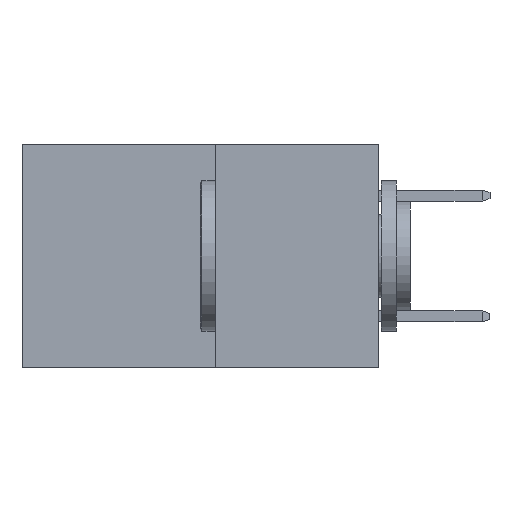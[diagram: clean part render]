
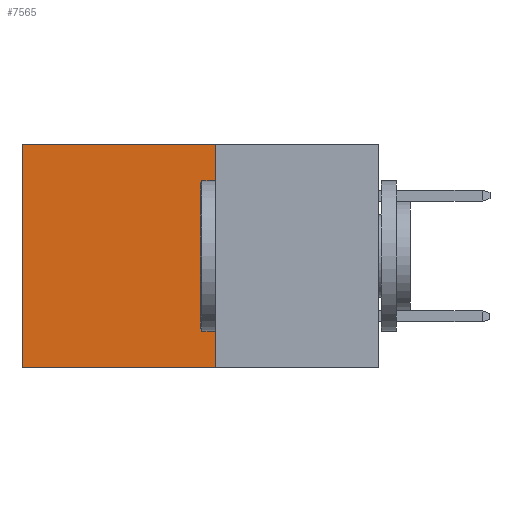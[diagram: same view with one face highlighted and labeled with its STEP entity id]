
A CAD part, left-side view. The second image highlights one B-rep face of the part: STEP entity #7565.
In plain terms, the highlighted planar face has unit normal (-1, 0, 0).
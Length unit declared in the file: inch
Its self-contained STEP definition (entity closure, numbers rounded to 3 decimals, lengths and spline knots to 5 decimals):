
#312 = AXIS2_PLACEMENT_3D ( 'NONE', #6959, #4473, #389 ) ;
#389 = DIRECTION ( 'NONE',  ( 0., 0., -1. ) ) ;
#523 = CARTESIAN_POINT ( 'NONE',  ( 0.277, 0.27, -0.37 ) ) ;
#697 = LINE ( 'NONE', #523, #2576 ) ;
#932 = DIRECTION ( 'NONE',  ( 0., 1., 0. ) ) ;
#1072 = ORIENTED_EDGE ( 'NONE', *, *, #3635, .F. ) ;
#1086 = CARTESIAN_POINT ( 'NONE',  ( 0.277, 0.27, -0.37 ) ) ;
#1194 = FACE_OUTER_BOUND ( 'NONE', #4344, .T. ) ;
#1295 = DIRECTION ( 'NONE',  ( 0., 0., -1. ) ) ;
#1376 = LINE ( 'NONE', #7771, #7960 ) ;
#2576 = VECTOR ( 'NONE', #1295, 39.37008 ) ;
#3232 = LINE ( 'NONE', #7819, #6601 ) ;
#3635 = EDGE_CURVE ( 'NONE', #4693, #6929, #8069, .T. ) ;
#3734 = CARTESIAN_POINT ( 'NONE',  ( 0.277, 0.59, 0. ) ) ;
#4002 = CARTESIAN_POINT ( 'NONE',  ( 0.277, 0.27, -0.37 ) ) ;
#4182 = ORIENTED_EDGE ( 'NONE', *, *, #4300, .T. ) ;
#4208 = CARTESIAN_POINT ( 'NONE',  ( 0.277, 0.59, -0.37 ) ) ;
#4300 = EDGE_CURVE ( 'NONE', #8153, #6929, #1376, .T. ) ;
#4344 = EDGE_LOOP ( 'NONE', ( #4182, #1072, #4581, #6261 ) ) ;
#4473 = DIRECTION ( 'NONE',  ( 1., 0., 0. ) ) ;
#4522 = EDGE_CURVE ( 'NONE', #6651, #8153, #3232, .T. ) ;
#4581 = ORIENTED_EDGE ( 'NONE', *, *, #8359, .F. ) ;
#4693 = VERTEX_POINT ( 'NONE', #4002 ) ;
#4746 = VECTOR ( 'NONE', #932, 39.37008 ) ;
#5865 = DIRECTION ( 'NONE',  ( 0., 1., 0. ) ) ;
#6261 = ORIENTED_EDGE ( 'NONE', *, *, #4522, .T. ) ;
#6601 = VECTOR ( 'NONE', #5865, 39.37008 ) ;
#6651 = VERTEX_POINT ( 'NONE', #6738 ) ;
#6738 = CARTESIAN_POINT ( 'NONE',  ( 0.277, 0.27, 0. ) ) ;
#6929 = VERTEX_POINT ( 'NONE', #4208 ) ;
#6959 = CARTESIAN_POINT ( 'NONE',  ( 0.277, 0.27, -0.37 ) ) ;
#7565 = ADVANCED_FACE ( 'NONE', ( #1194 ), #8202, .F. ) ;
#7771 = CARTESIAN_POINT ( 'NONE',  ( 0.277, 0.59, -0.37 ) ) ;
#7819 = CARTESIAN_POINT ( 'NONE',  ( 0.277, 0.27, 0. ) ) ;
#7960 = VECTOR ( 'NONE', #8407, 39.37008 ) ;
#8069 = LINE ( 'NONE', #1086, #4746 ) ;
#8153 = VERTEX_POINT ( 'NONE', #3734 ) ;
#8202 = PLANE ( 'NONE',  #312 ) ;
#8359 = EDGE_CURVE ( 'NONE', #6651, #4693, #697, .T. ) ;
#8407 = DIRECTION ( 'NONE',  ( 0., 0., -1. ) ) ;
